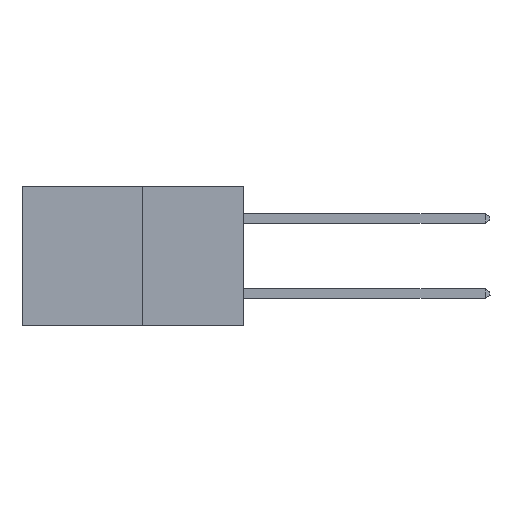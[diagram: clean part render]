
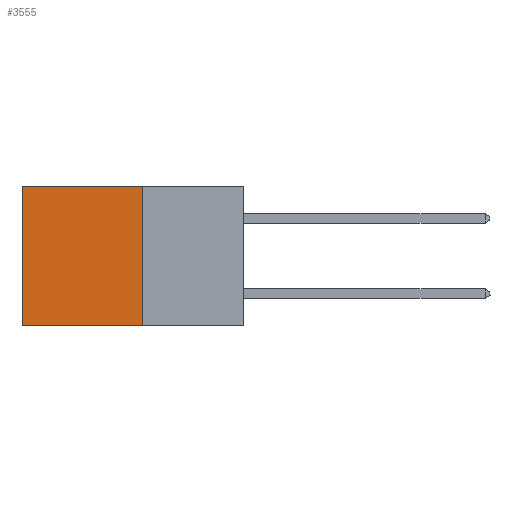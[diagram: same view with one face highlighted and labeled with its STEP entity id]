
A CAD part, left-side view. The second image highlights one B-rep face of the part: STEP entity #3555.
In plain terms, the highlighted planar face has unit normal (-1, 0, 0).
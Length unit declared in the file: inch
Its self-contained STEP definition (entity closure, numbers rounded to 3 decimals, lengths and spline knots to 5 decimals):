
#442 = LINE ( 'NONE', #6972, #3747 ) ;
#474 = ORIENTED_EDGE ( 'NONE', *, *, #5940, .F. ) ;
#492 = CARTESIAN_POINT ( 'NONE',  ( 0.277, 0.27, -0.37 ) ) ;
#526 = CARTESIAN_POINT ( 'NONE',  ( 0.277, 0.27, 0. ) ) ;
#562 = VERTEX_POINT ( 'NONE', #7862 ) ;
#566 = ORIENTED_EDGE ( 'NONE', *, *, #7053, .T. ) ;
#587 = VECTOR ( 'NONE', #5660, 39.37008 ) ;
#683 = ORIENTED_EDGE ( 'NONE', *, *, #3343, .T. ) ;
#945 = VERTEX_POINT ( 'NONE', #6746 ) ;
#1254 = CARTESIAN_POINT ( 'NONE',  ( 0.277, 0.27, -0.37 ) ) ;
#1892 = PLANE ( 'NONE',  #2967 ) ;
#1926 = DIRECTION ( 'NONE',  ( 0., 1., 0. ) ) ;
#2485 = DIRECTION ( 'NONE',  ( 0., 0., -1. ) ) ;
#2627 = DIRECTION ( 'NONE',  ( 1., 0., 0. ) ) ;
#2770 = ORIENTED_EDGE ( 'NONE', *, *, #8555, .F. ) ;
#2928 = VECTOR ( 'NONE', #1926, 39.37008 ) ;
#2959 = VERTEX_POINT ( 'NONE', #5579 ) ;
#2967 = AXIS2_PLACEMENT_3D ( 'NONE', #3617, #2627, #2485 ) ;
#3123 = LINE ( 'NONE', #1254, #2928 ) ;
#3343 = EDGE_CURVE ( 'NONE', #562, #6018, #5617, .T. ) ;
#3555 = ADVANCED_FACE ( 'NONE', ( #7260 ), #1892, .F. ) ;
#3617 = CARTESIAN_POINT ( 'NONE',  ( 0.277, 0.27, -0.37 ) ) ;
#3747 = VECTOR ( 'NONE', #7644, 39.37008 ) ;
#4456 = DIRECTION ( 'NONE',  ( 0., 0., -1. ) ) ;
#4538 = CARTESIAN_POINT ( 'NONE',  ( 0.277, 0.59, 0. ) ) ;
#5579 = CARTESIAN_POINT ( 'NONE',  ( 0.277, 0.59, -0.37 ) ) ;
#5617 = LINE ( 'NONE', #526, #587 ) ;
#5660 = DIRECTION ( 'NONE',  ( 0., 1., 0. ) ) ;
#5753 = EDGE_LOOP ( 'NONE', ( #566, #2770, #474, #683 ) ) ;
#5940 = EDGE_CURVE ( 'NONE', #562, #945, #7662, .T. ) ;
#6018 = VERTEX_POINT ( 'NONE', #4538 ) ;
#6746 = CARTESIAN_POINT ( 'NONE',  ( 0.277, 0.27, -0.37 ) ) ;
#6972 = CARTESIAN_POINT ( 'NONE',  ( 0.277, 0.59, -0.37 ) ) ;
#7053 = EDGE_CURVE ( 'NONE', #6018, #2959, #442, .T. ) ;
#7234 = VECTOR ( 'NONE', #4456, 39.37008 ) ;
#7260 = FACE_OUTER_BOUND ( 'NONE', #5753, .T. ) ;
#7644 = DIRECTION ( 'NONE',  ( 0., 0., -1. ) ) ;
#7662 = LINE ( 'NONE', #492, #7234 ) ;
#7862 = CARTESIAN_POINT ( 'NONE',  ( 0.277, 0.27, 0. ) ) ;
#8555 = EDGE_CURVE ( 'NONE', #945, #2959, #3123, .T. ) ;
